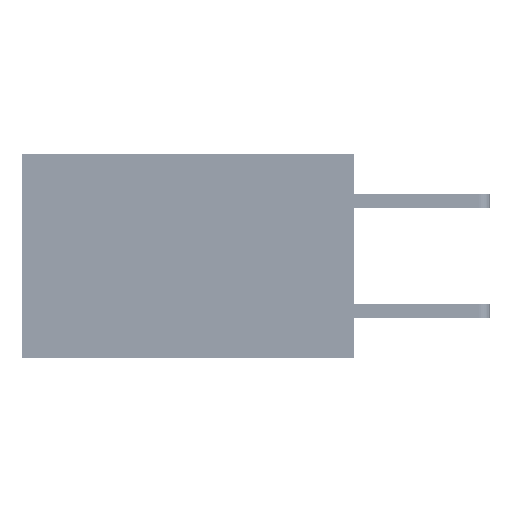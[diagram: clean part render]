
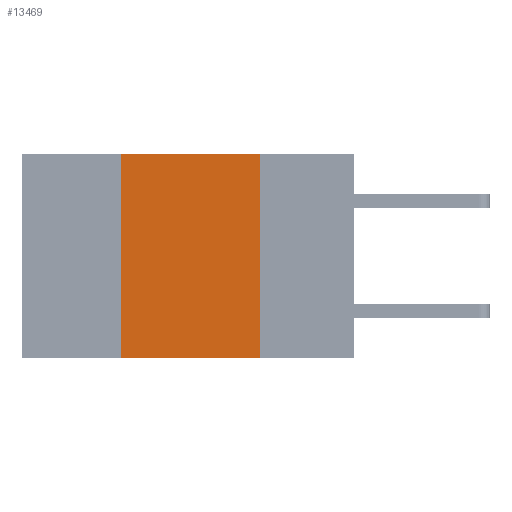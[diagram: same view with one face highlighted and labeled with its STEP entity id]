
A CAD part, left-side view. The second image highlights one B-rep face of the part: STEP entity #13469.
In plain terms, the highlighted planar face has unit normal (-1, 0, 0).
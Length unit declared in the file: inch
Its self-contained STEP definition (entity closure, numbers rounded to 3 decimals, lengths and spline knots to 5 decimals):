
#601 = CARTESIAN_POINT ( 'NONE',  ( 0., 0.42, 0. ) ) ;
#1308 = VERTEX_POINT ( 'NONE', #601 ) ;
#1922 = EDGE_CURVE ( 'NONE', #1308, #30587, #15627, .T. ) ;
#2003 = FACE_OUTER_BOUND ( 'NONE', #38918, .T. ) ;
#2654 = VECTOR ( 'NONE', #8715, 39.37008 ) ;
#4574 = DIRECTION ( 'NONE',  ( 0., 0., -1. ) ) ;
#6496 = DIRECTION ( 'NONE',  ( 0., 0., -1. ) ) ;
#6781 = CARTESIAN_POINT ( 'NONE',  ( 0., 0.6, 0. ) ) ;
#7506 = VERTEX_POINT ( 'NONE', #39161 ) ;
#7560 = CARTESIAN_POINT ( 'NONE',  ( 0., 0.42, 0. ) ) ;
#8715 = DIRECTION ( 'NONE',  ( 0., -1., 0. ) ) ;
#11179 = CARTESIAN_POINT ( 'NONE',  ( 0., 0.6, 0. ) ) ;
#11851 = LINE ( 'NONE', #24926, #2654 ) ;
#11922 = EDGE_CURVE ( 'NONE', #7506, #38431, #11851, .T. ) ;
#13469 = ADVANCED_FACE ( 'NONE', ( #2003 ), #35782, .F. ) ;
#14192 = DIRECTION ( 'NONE',  ( 0., -1., 0. ) ) ;
#15193 = CARTESIAN_POINT ( 'NONE',  ( 0., 0.17, 0. ) ) ;
#15627 = LINE ( 'NONE', #11179, #40533 ) ;
#17816 = ORIENTED_EDGE ( 'NONE', *, *, #34196, .F. ) ;
#21795 = ORIENTED_EDGE ( 'NONE', *, *, #30421, .F. ) ;
#24634 = LINE ( 'NONE', #33281, #33251 ) ;
#24926 = CARTESIAN_POINT ( 'NONE',  ( 0., 0.6, -0.37 ) ) ;
#25970 = DIRECTION ( 'NONE',  ( 1., 0., 0. ) ) ;
#30421 = EDGE_CURVE ( 'NONE', #30587, #38431, #24634, .T. ) ;
#30587 = VERTEX_POINT ( 'NONE', #15193 ) ;
#31078 = ORIENTED_EDGE ( 'NONE', *, *, #1922, .F. ) ;
#32230 = ORIENTED_EDGE ( 'NONE', *, *, #11922, .T. ) ;
#33251 = VECTOR ( 'NONE', #4574, 39.37008 ) ;
#33281 = CARTESIAN_POINT ( 'NONE',  ( 0., 0.17, 0. ) ) ;
#34196 = EDGE_CURVE ( 'NONE', #7506, #1308, #38945, .T. ) ;
#35211 = CARTESIAN_POINT ( 'NONE',  ( 0., 0.17, -0.37 ) ) ;
#35782 = PLANE ( 'NONE',  #37826 ) ;
#37826 = AXIS2_PLACEMENT_3D ( 'NONE', #6781, #25970, #6496 ) ;
#37912 = VECTOR ( 'NONE', #40376, 39.37008 ) ;
#38431 = VERTEX_POINT ( 'NONE', #35211 ) ;
#38918 = EDGE_LOOP ( 'NONE', ( #21795, #31078, #17816, #32230 ) ) ;
#38945 = LINE ( 'NONE', #7560, #37912 ) ;
#39161 = CARTESIAN_POINT ( 'NONE',  ( 0., 0.42, -0.37 ) ) ;
#40376 = DIRECTION ( 'NONE',  ( 0., 0., 1. ) ) ;
#40533 = VECTOR ( 'NONE', #14192, 39.37008 ) ;
